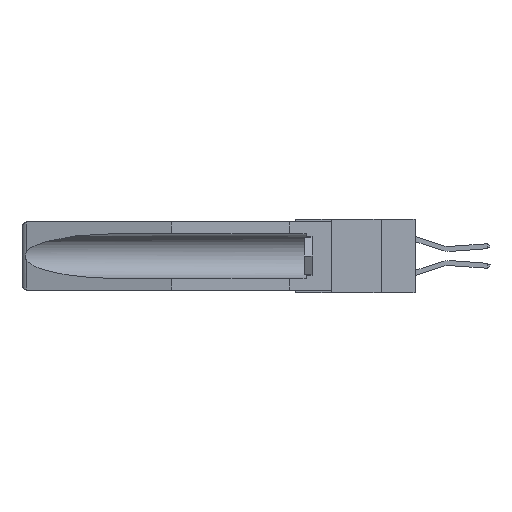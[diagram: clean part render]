
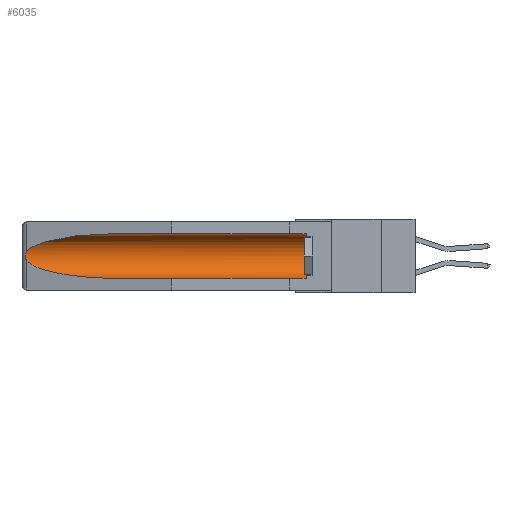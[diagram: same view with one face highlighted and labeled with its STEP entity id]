
A CAD part, left-side view. The second image highlights one B-rep face of the part: STEP entity #6035.
In plain terms, the highlighted cylindrical face has radius 2.857 mm (diameter 5.715 mm), a partial arc.
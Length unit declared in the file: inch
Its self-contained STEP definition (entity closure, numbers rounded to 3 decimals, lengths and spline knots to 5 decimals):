
#74 = VERTEX_POINT ( 'NONE', #6936 ) ;
#747 = AXIS2_PLACEMENT_3D ( 'NONE', #7291, #10094, #20845 ) ;
#1677 = CARTESIAN_POINT ( 'NONE',  ( 0.26537, 1.52718, -0.19328 ) ) ;
#2868 = LINE ( 'NONE', #20369, #7292 ) ;
#3113 = CARTESIAN_POINT ( 'NONE',  ( 0.155, 1.07973, -0.059 ) ) ;
#3142 = CARTESIAN_POINT ( 'NONE',  ( 0.25451, 1.48313, -0.09465 ) ) ;
#3154 = EDGE_CURVE ( 'NONE', #11772, #19490, #12434, .T. ) ;
#3395 = FACE_OUTER_BOUND ( 'NONE', #26359, .T. ) ;
#3901 = CARTESIAN_POINT ( 'NONE',  ( 0.2675, 1.53308, -0.17534 ) ) ;
#4629 = CARTESIAN_POINT ( 'NONE',  ( 0.155, 1.07973, -0.284 ) ) ;
#4756 = LINE ( 'NONE', #33386, #19745 ) ;
#5458 = CARTESIAN_POINT ( 'NONE',  ( 0.21114, 1.30732, -0.059 ) ) ;
#6035 = ADVANCED_FACE ( 'NONE', ( #3395 ), #30131, .F. ) ;
#6936 = CARTESIAN_POINT ( 'NONE',  ( 0.155, 0.126, -0.059 ) ) ;
#7059 = ORIENTED_EDGE ( 'NONE', *, *, #17776, .F. ) ;
#7139 = CARTESIAN_POINT ( 'NONE',  ( 0.21114, 1.30732, -0.284 ) ) ;
#7291 = CARTESIAN_POINT ( 'NONE',  ( 0.155, 0.126, -0.1715 ) ) ;
#7292 = VECTOR ( 'NONE', #23173, 39.37008 ) ;
#7471 = ORIENTED_EDGE ( 'NONE', *, *, #3154, .T. ) ;
#7942 = EDGE_CURVE ( 'NONE', #28357, #74, #15394, .T. ) ;
#8464 = ORIENTED_EDGE ( 'NONE', *, *, #26748, .T. ) ;
#9037 = CARTESIAN_POINT ( 'NONE',  ( 0.26537, 1.52718, -0.14972 ) ) ;
#9065 = DIRECTION ( 'NONE',  ( 0., 1., 0. ) ) ;
#9542 = CARTESIAN_POINT ( 'NONE',  ( 0.26537, 1.52718, -0.14972 ) ) ;
#9577 = VERTEX_POINT ( 'NONE', #3113 ) ;
#10094 = DIRECTION ( 'NONE',  ( 0., -1., 0. ) ) ;
#10822 = EDGE_CURVE ( 'NONE', #9577, #22388, #20500, .T. ) ;
#11073 = CARTESIAN_POINT ( 'NONE',  ( 0.26537, 1.52718, -0.19328 ) ) ;
#11772 = VERTEX_POINT ( 'NONE', #11073 ) ;
#11830 = CARTESIAN_POINT ( 'NONE',  ( 0.2673, 1.53269, -0.17917 ) ) ;
#11952 = CARTESIAN_POINT ( 'NONE',  ( 0.26654, 1.53092, -0.15636 ) ) ;
#12434 =( BOUNDED_CURVE ( )  B_SPLINE_CURVE ( 3, ( #1677, #23157, #7139, #34153 ),
 .UNSPECIFIED., .F., .F. ) 
 B_SPLINE_CURVE_WITH_KNOTS ( ( 4, 4 ),
 ( 0.1948, 1.5708 ),
 .UNSPECIFIED. ) 
 CURVE ( )  GEOMETRIC_REPRESENTATION_ITEM ( )  RATIONAL_B_SPLINE_CURVE ( ( 1., 0.848, 0.848, 1. ) ) 
 REPRESENTATION_ITEM ( '' )  );
#13090 = CARTESIAN_POINT ( 'NONE',  ( 0.155, 1.07973, -0.059 ) ) ;
#13871 = EDGE_CURVE ( 'NONE', #74, #9577, #2868, .T. ) ;
#14195 = CARTESIAN_POINT ( 'NONE',  ( 0.26537, 1.52718, -0.19328 ) ) ;
#14368 = DIRECTION ( 'NONE',  ( 0., 1., 0. ) ) ;
#14481 = CARTESIAN_POINT ( 'NONE',  ( 0.155, -0.30754, -0.1715 ) ) ;
#14660 = CARTESIAN_POINT ( 'NONE',  ( 0.26597, 1.52961, -0.15275 ) ) ;
#15074 = DIRECTION ( 'NONE',  ( 0., 0., 1. ) ) ;
#15394 = CIRCLE ( 'NONE', #747, 0.1125 ) ;
#16878 = CARTESIAN_POINT ( 'NONE',  ( 0.2673, 1.5327, -0.16383 ) ) ;
#17340 = CARTESIAN_POINT ( 'NONE',  ( 0.26655, 1.53094, -0.18657 ) ) ;
#17776 = EDGE_CURVE ( 'NONE', #28357, #19490, #4756, .T. ) ;
#19490 = VERTEX_POINT ( 'NONE', #4629 ) ;
#19745 = VECTOR ( 'NONE', #9065, 39.37008 ) ;
#20369 = CARTESIAN_POINT ( 'NONE',  ( 0.155, -0.30754, -0.059 ) ) ;
#20500 =( BOUNDED_CURVE ( )  B_SPLINE_CURVE ( 3, ( #13090, #5458, #3142, #32700 ),
 .UNSPECIFIED., .F., .F. ) 
 B_SPLINE_CURVE_WITH_KNOTS ( ( 4, 4 ),
 ( 4.71239, 6.08839 ),
 .UNSPECIFIED. ) 
 CURVE ( )  GEOMETRIC_REPRESENTATION_ITEM ( )  RATIONAL_B_SPLINE_CURVE ( ( 1., 0.848, 0.848, 1. ) ) 
 REPRESENTATION_ITEM ( '' )  );
#20845 = DIRECTION ( 'NONE',  ( 0., 0., 1. ) ) ;
#22141 = ORIENTED_EDGE ( 'NONE', *, *, #13871, .T. ) ;
#22359 = CARTESIAN_POINT ( 'NONE',  ( 0.2675, 1.53308, -0.16763 ) ) ;
#22388 = VERTEX_POINT ( 'NONE', #9542 ) ;
#23157 = CARTESIAN_POINT ( 'NONE',  ( 0.25451, 1.48313, -0.24835 ) ) ;
#23173 = DIRECTION ( 'NONE',  ( 0., 1., 0. ) ) ;
#24621 = ORIENTED_EDGE ( 'NONE', *, *, #7942, .T. ) ;
#25261 = AXIS2_PLACEMENT_3D ( 'NONE', #14481, #14368, #15074 ) ;
#26359 = EDGE_LOOP ( 'NONE', ( #30490, #8464, #7471, #7059, #24621, #22141 ) ) ;
#26748 = EDGE_CURVE ( 'NONE', #22388, #11772, #31450, .T. ) ;
#28357 = VERTEX_POINT ( 'NONE', #30549 ) ;
#30131 = CYLINDRICAL_SURFACE ( 'NONE', #25261, 0.1125 ) ;
#30438 = CARTESIAN_POINT ( 'NONE',  ( 0.26597, 1.5296, -0.19026 ) ) ;
#30490 = ORIENTED_EDGE ( 'NONE', *, *, #10822, .T. ) ;
#30549 = CARTESIAN_POINT ( 'NONE',  ( 0.155, 0.126, -0.284 ) ) ;
#31450 = B_SPLINE_CURVE_WITH_KNOTS ( 'NONE', 3,
 ( #9037, #14660, #11952, #16878, #22359, #3901, #11830, #17340, #30438, #14195 ),
 .UNSPECIFIED., .F., .F.,
 ( 4, 2, 2, 2, 4 ),
 ( 0., 0.00029, 0.00058, 0.00087, 0.00117 ),
 .UNSPECIFIED. ) ;
#32700 = CARTESIAN_POINT ( 'NONE',  ( 0.26537, 1.52718, -0.14972 ) ) ;
#33386 = CARTESIAN_POINT ( 'NONE',  ( 0.155, -0.30754, -0.284 ) ) ;
#34153 = CARTESIAN_POINT ( 'NONE',  ( 0.155, 1.07973, -0.284 ) ) ;
